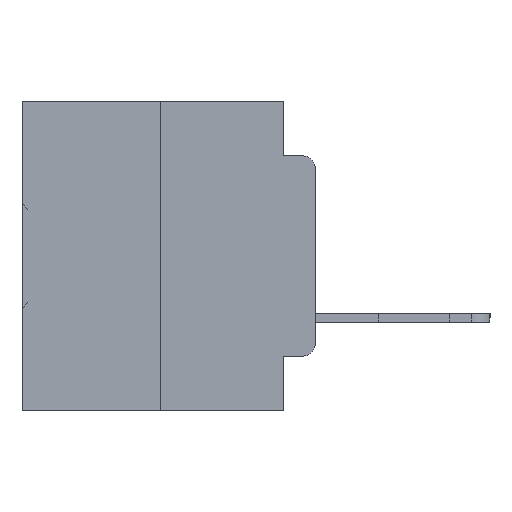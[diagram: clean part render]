
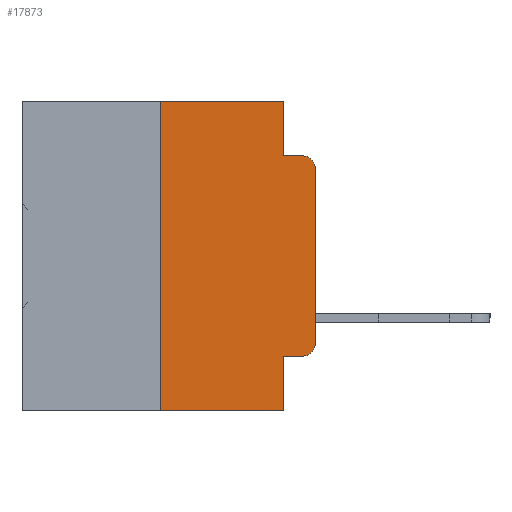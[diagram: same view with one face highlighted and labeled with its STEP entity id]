
A CAD part, left-side view. The second image highlights one B-rep face of the part: STEP entity #17873.
In plain terms, the highlighted planar face has unit normal (-1, 0, 0).
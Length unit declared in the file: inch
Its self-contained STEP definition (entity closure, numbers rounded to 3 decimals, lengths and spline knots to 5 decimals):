
#125 = LINE ( 'NONE', #7797, #27721 ) ;
#129 = ORIENTED_EDGE ( 'NONE', *, *, #16865, .T. ) ;
#429 = CARTESIAN_POINT ( 'NONE',  ( 0., 0.051, -0.0885 ) ) ;
#579 = DIRECTION ( 'NONE',  ( 0., 0., 1. ) ) ;
#1009 = VECTOR ( 'NONE', #24556, 39.37008 ) ;
#1704 = CARTESIAN_POINT ( 'NONE',  ( 0., 0.02, -0.3915 ) ) ;
#1716 = LINE ( 'NONE', #1863, #8240 ) ;
#1863 = CARTESIAN_POINT ( 'NONE',  ( 0., 0.051, -0.4115 ) ) ;
#2012 = AXIS2_PLACEMENT_3D ( 'NONE', #4137, #22820, #6948 ) ;
#3592 = VERTEX_POINT ( 'NONE', #20524 ) ;
#3689 = VERTEX_POINT ( 'NONE', #10097 ) ;
#4137 = CARTESIAN_POINT ( 'NONE',  ( 0., 0.02, -0.1085 ) ) ;
#4522 = DIRECTION ( 'NONE',  ( 0., 0., -1. ) ) ;
#4935 = EDGE_CURVE ( 'NONE', #31089, #22534, #14669, .T. ) ;
#4989 = EDGE_CURVE ( 'NONE', #34101, #8230, #27675, .T. ) ;
#5665 = ORIENTED_EDGE ( 'NONE', *, *, #9296, .T. ) ;
#6012 = DIRECTION ( 'NONE',  ( 0., -1., 0. ) ) ;
#6254 = CARTESIAN_POINT ( 'NONE',  ( 0., 0.473, 0. ) ) ;
#6640 = ORIENTED_EDGE ( 'NONE', *, *, #18161, .F. ) ;
#6948 = DIRECTION ( 'NONE',  ( 0., 0., -1. ) ) ;
#7012 = CARTESIAN_POINT ( 'NONE',  ( 0., 0.02, -0.0885 ) ) ;
#7797 = CARTESIAN_POINT ( 'NONE',  ( 0., 0.25, 0. ) ) ;
#8230 = VERTEX_POINT ( 'NONE', #20551 ) ;
#8240 = VECTOR ( 'NONE', #20716, 39.37008 ) ;
#8263 = ORIENTED_EDGE ( 'NONE', *, *, #19330, .F. ) ;
#9121 = CARTESIAN_POINT ( 'NONE',  ( 0., 0.051, -0.0885 ) ) ;
#9201 = VECTOR ( 'NONE', #6012, 39.37008 ) ;
#9296 = EDGE_CURVE ( 'NONE', #14360, #28671, #1716, .T. ) ;
#10028 = LINE ( 'NONE', #19309, #9201 ) ;
#10056 = ORIENTED_EDGE ( 'NONE', *, *, #32553, .T. ) ;
#10097 = CARTESIAN_POINT ( 'NONE',  ( 0., 0., -0.1085 ) ) ;
#12009 = EDGE_CURVE ( 'NONE', #3592, #3689, #17868, .T. ) ;
#12210 = ORIENTED_EDGE ( 'NONE', *, *, #16431, .F. ) ;
#13176 = DIRECTION ( 'NONE',  ( 0., 0., -1. ) ) ;
#13391 = CIRCLE ( 'NONE', #2012, 0.02 ) ;
#14287 = ORIENTED_EDGE ( 'NONE', *, *, #28538, .F. ) ;
#14360 = VERTEX_POINT ( 'NONE', #17062 ) ;
#14669 = LINE ( 'NONE', #429, #1009 ) ;
#16407 = ORIENTED_EDGE ( 'NONE', *, *, #4989, .T. ) ;
#16431 = EDGE_CURVE ( 'NONE', #14360, #8230, #21247, .T. ) ;
#16865 = EDGE_CURVE ( 'NONE', #3689, #22534, #13391, .T. ) ;
#17008 = DIRECTION ( 'NONE',  ( 0., 0., -1. ) ) ;
#17062 = CARTESIAN_POINT ( 'NONE',  ( 0., 0.051, -0.4115 ) ) ;
#17095 = CARTESIAN_POINT ( 'NONE',  ( 0., 0.473, -0.5 ) ) ;
#17443 = CIRCLE ( 'NONE', #32092, 0.02 ) ;
#17868 = LINE ( 'NONE', #19530, #29954 ) ;
#17873 = ADVANCED_FACE ( 'NONE', ( #24596 ), #29832, .F. ) ;
#18161 = EDGE_CURVE ( 'NONE', #34101, #26142, #125, .T. ) ;
#18167 = CARTESIAN_POINT ( 'NONE',  ( 0., 0.02, -0.4115 ) ) ;
#18342 = DIRECTION ( 'NONE',  ( 0., 0., 1. ) ) ;
#19309 = CARTESIAN_POINT ( 'NONE',  ( 0., 0.473, 0. ) ) ;
#19330 = EDGE_CURVE ( 'NONE', #26142, #19743, #10028, .T. ) ;
#19530 = CARTESIAN_POINT ( 'NONE',  ( 0., 0., 0. ) ) ;
#19632 = DIRECTION ( 'NONE',  ( 0., -1., 0. ) ) ;
#19743 = VERTEX_POINT ( 'NONE', #31435 ) ;
#19748 = ORIENTED_EDGE ( 'NONE', *, *, #12009, .T. ) ;
#20021 = VECTOR ( 'NONE', #19632, 39.37008 ) ;
#20524 = CARTESIAN_POINT ( 'NONE',  ( 0., 0., -0.3915 ) ) ;
#20551 = CARTESIAN_POINT ( 'NONE',  ( 0., 0.051, -0.5 ) ) ;
#20562 = DIRECTION ( 'NONE',  ( -1., 0., 0. ) ) ;
#20716 = DIRECTION ( 'NONE',  ( 0., -1., 0. ) ) ;
#20967 = AXIS2_PLACEMENT_3D ( 'NONE', #6254, #32378, #17008 ) ;
#21247 = LINE ( 'NONE', #28721, #27295 ) ;
#22167 = CARTESIAN_POINT ( 'NONE',  ( 0., 0.25, -0.5 ) ) ;
#22534 = VERTEX_POINT ( 'NONE', #7012 ) ;
#22820 = DIRECTION ( 'NONE',  ( -1., 0., 0. ) ) ;
#24171 = ORIENTED_EDGE ( 'NONE', *, *, #4935, .F. ) ;
#24556 = DIRECTION ( 'NONE',  ( 0., -1., 0. ) ) ;
#24596 = FACE_OUTER_BOUND ( 'NONE', #32940, .T. ) ;
#25510 = DIRECTION ( 'NONE',  ( 0., 0., -1. ) ) ;
#26142 = VERTEX_POINT ( 'NONE', #31962 ) ;
#27295 = VECTOR ( 'NONE', #13176, 39.37008 ) ;
#27675 = LINE ( 'NONE', #17095, #20021 ) ;
#27721 = VECTOR ( 'NONE', #18342, 39.37008 ) ;
#27737 = VECTOR ( 'NONE', #25510, 39.37008 ) ;
#28513 = LINE ( 'NONE', #33080, #27737 ) ;
#28538 = EDGE_CURVE ( 'NONE', #19743, #31089, #28513, .T. ) ;
#28671 = VERTEX_POINT ( 'NONE', #18167 ) ;
#28721 = CARTESIAN_POINT ( 'NONE',  ( 0., 0.051, 0. ) ) ;
#29832 = PLANE ( 'NONE',  #20967 ) ;
#29954 = VECTOR ( 'NONE', #579, 39.37008 ) ;
#31089 = VERTEX_POINT ( 'NONE', #9121 ) ;
#31435 = CARTESIAN_POINT ( 'NONE',  ( 0., 0.051, 0. ) ) ;
#31962 = CARTESIAN_POINT ( 'NONE',  ( 0., 0.25, 0. ) ) ;
#32092 = AXIS2_PLACEMENT_3D ( 'NONE', #1704, #20562, #4522 ) ;
#32378 = DIRECTION ( 'NONE',  ( 1., 0., 0. ) ) ;
#32553 = EDGE_CURVE ( 'NONE', #28671, #3592, #17443, .T. ) ;
#32940 = EDGE_LOOP ( 'NONE', ( #19748, #129, #24171, #14287, #8263, #6640, #16407, #12210, #5665, #10056 ) ) ;
#33080 = CARTESIAN_POINT ( 'NONE',  ( 0., 0.051, 0. ) ) ;
#34101 = VERTEX_POINT ( 'NONE', #22167 ) ;
